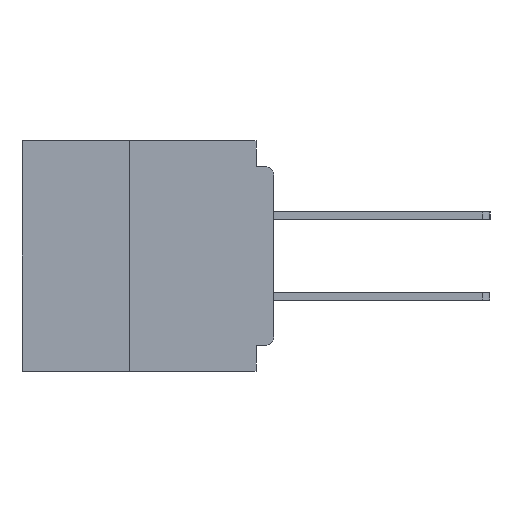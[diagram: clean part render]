
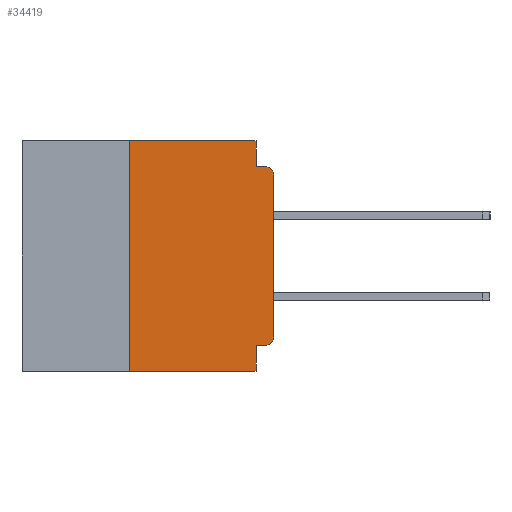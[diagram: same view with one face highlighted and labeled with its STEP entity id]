
A CAD part, left-side view. The second image highlights one B-rep face of the part: STEP entity #34419.
In plain terms, the highlighted planar face has unit normal (-1, 0, 0).
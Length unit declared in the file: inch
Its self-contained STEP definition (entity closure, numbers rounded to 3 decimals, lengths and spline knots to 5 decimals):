
#31 = VECTOR ( 'NONE', #66891, 39.37008 ) ;
#384 = VERTEX_POINT ( 'NONE', #27047 ) ;
#1747 = VERTEX_POINT ( 'NONE', #54699 ) ;
#2224 = DIRECTION ( 'NONE',  ( 0., 0., -1. ) ) ;
#2491 = LINE ( 'NONE', #56251, #28710 ) ;
#3141 = CARTESIAN_POINT ( 'NONE',  ( 0., 0.25, -0.4 ) ) ;
#3195 = DIRECTION ( 'NONE',  ( -1., 0., 0. ) ) ;
#5137 = CARTESIAN_POINT ( 'NONE',  ( 0., 0.031, -0.4 ) ) ;
#6063 = CARTESIAN_POINT ( 'NONE',  ( 0., 0., -0.355 ) ) ;
#6633 = DIRECTION ( 'NONE',  ( 0., -1., 0. ) ) ;
#8123 = EDGE_CURVE ( 'NONE', #63116, #41610, #60506, .T. ) ;
#8308 = ORIENTED_EDGE ( 'NONE', *, *, #26199, .F. ) ;
#9129 = VERTEX_POINT ( 'NONE', #14503 ) ;
#11056 = CIRCLE ( 'NONE', #36068, 0.015 ) ;
#11077 = LINE ( 'NONE', #55611, #64418 ) ;
#11372 = DIRECTION ( 'NONE',  ( 0., 1., 0. ) ) ;
#11818 = CARTESIAN_POINT ( 'NONE',  ( 0., 0.031, -0.4 ) ) ;
#12473 = CIRCLE ( 'NONE', #44600, 0.015 ) ;
#12802 = VECTOR ( 'NONE', #41342, 39.37008 ) ;
#13586 = ORIENTED_EDGE ( 'NONE', *, *, #39826, .F. ) ;
#14503 = CARTESIAN_POINT ( 'NONE',  ( 0., 0., -0.34 ) ) ;
#15498 = DIRECTION ( 'NONE',  ( 0., -1., 0. ) ) ;
#16225 = LINE ( 'NONE', #37921, #40651 ) ;
#16384 = ORIENTED_EDGE ( 'NONE', *, *, #24180, .T. ) ;
#16412 = VECTOR ( 'NONE', #15498, 39.37008 ) ;
#17131 = EDGE_LOOP ( 'NONE', ( #53732, #59925, #13586, #56914, #32302, #30323, #16384, #34218, #8308, #52899 ) ) ;
#19761 = DIRECTION ( 'NONE',  ( 0., 0., 1. ) ) ;
#20773 = EDGE_CURVE ( 'NONE', #53980, #32496, #11077, .T. ) ;
#24178 = VERTEX_POINT ( 'NONE', #46769 ) ;
#24180 = EDGE_CURVE ( 'NONE', #53980, #41610, #30294, .T. ) ;
#24977 = PLANE ( 'NONE',  #39790 ) ;
#26199 = EDGE_CURVE ( 'NONE', #1747, #63116, #34080, .T. ) ;
#27047 = CARTESIAN_POINT ( 'NONE',  ( 0., 0., -0.06 ) ) ;
#28710 = VECTOR ( 'NONE', #61418, 39.37008 ) ;
#30294 = LINE ( 'NONE', #67096, #16412 ) ;
#30323 = ORIENTED_EDGE ( 'NONE', *, *, #20773, .F. ) ;
#30913 = CARTESIAN_POINT ( 'NONE',  ( 0., 0., 0. ) ) ;
#31245 = VERTEX_POINT ( 'NONE', #44034 ) ;
#32302 = ORIENTED_EDGE ( 'NONE', *, *, #44578, .F. ) ;
#32496 = VERTEX_POINT ( 'NONE', #35422 ) ;
#32910 = EDGE_CURVE ( 'NONE', #1747, #9129, #11056, .T. ) ;
#33536 = DIRECTION ( 'NONE',  ( -1., 0., 0. ) ) ;
#33769 = CARTESIAN_POINT ( 'NONE',  ( 0., 0.015, -0.045 ) ) ;
#34080 = LINE ( 'NONE', #6063, #58157 ) ;
#34218 = ORIENTED_EDGE ( 'NONE', *, *, #8123, .F. ) ;
#34419 = ADVANCED_FACE ( 'NONE', ( #49069 ), #24977, .F. ) ;
#34508 = CARTESIAN_POINT ( 'NONE',  ( 0., 0.015, -0.06 ) ) ;
#35411 = DIRECTION ( 'NONE',  ( 0., 0., -1. ) ) ;
#35422 = CARTESIAN_POINT ( 'NONE',  ( 0., 0.25, 0. ) ) ;
#35795 = EDGE_CURVE ( 'NONE', #24178, #31245, #65696, .T. ) ;
#36068 = AXIS2_PLACEMENT_3D ( 'NONE', #64267, #33536, #2224 ) ;
#36228 = CARTESIAN_POINT ( 'NONE',  ( 0., 0.031, 0. ) ) ;
#37822 = DIRECTION ( 'NONE',  ( 0., 0., -1. ) ) ;
#37921 = CARTESIAN_POINT ( 'NONE',  ( 0., 0., -0.045 ) ) ;
#39737 = DIRECTION ( 'NONE',  ( 0., 0., -1. ) ) ;
#39790 = AXIS2_PLACEMENT_3D ( 'NONE', #60965, #66092, #35411 ) ;
#39826 = EDGE_CURVE ( 'NONE', #31245, #44933, #16225, .T. ) ;
#40523 = LINE ( 'NONE', #30913, #12802 ) ;
#40651 = VECTOR ( 'NONE', #6633, 39.37008 ) ;
#41342 = DIRECTION ( 'NONE',  ( 0., 0., 1. ) ) ;
#41610 = VERTEX_POINT ( 'NONE', #5137 ) ;
#44034 = CARTESIAN_POINT ( 'NONE',  ( 0., 0.031, -0.045 ) ) ;
#44578 = EDGE_CURVE ( 'NONE', #32496, #24178, #2491, .T. ) ;
#44600 = AXIS2_PLACEMENT_3D ( 'NONE', #34508, #3195, #39737 ) ;
#44933 = VERTEX_POINT ( 'NONE', #33769 ) ;
#46316 = EDGE_CURVE ( 'NONE', #384, #44933, #12473, .T. ) ;
#46769 = CARTESIAN_POINT ( 'NONE',  ( 0., 0.031, 0. ) ) ;
#49069 = FACE_OUTER_BOUND ( 'NONE', #17131, .T. ) ;
#49655 = EDGE_CURVE ( 'NONE', #9129, #384, #40523, .T. ) ;
#52899 = ORIENTED_EDGE ( 'NONE', *, *, #32910, .T. ) ;
#53732 = ORIENTED_EDGE ( 'NONE', *, *, #49655, .T. ) ;
#53859 = CARTESIAN_POINT ( 'NONE',  ( 0., 0.031, -0.355 ) ) ;
#53980 = VERTEX_POINT ( 'NONE', #3141 ) ;
#54699 = CARTESIAN_POINT ( 'NONE',  ( 0., 0.015, -0.355 ) ) ;
#55611 = CARTESIAN_POINT ( 'NONE',  ( 0., 0.25, -0.4 ) ) ;
#56251 = CARTESIAN_POINT ( 'NONE',  ( 0., 0.437, 0. ) ) ;
#56914 = ORIENTED_EDGE ( 'NONE', *, *, #35795, .F. ) ;
#57266 = VECTOR ( 'NONE', #37822, 39.37008 ) ;
#58157 = VECTOR ( 'NONE', #11372, 39.37008 ) ;
#59925 = ORIENTED_EDGE ( 'NONE', *, *, #46316, .T. ) ;
#60506 = LINE ( 'NONE', #11818, #57266 ) ;
#60965 = CARTESIAN_POINT ( 'NONE',  ( 0., 0.437, 0. ) ) ;
#61418 = DIRECTION ( 'NONE',  ( 0., -1., 0. ) ) ;
#63116 = VERTEX_POINT ( 'NONE', #53859 ) ;
#64267 = CARTESIAN_POINT ( 'NONE',  ( 0., 0.015, -0.34 ) ) ;
#64418 = VECTOR ( 'NONE', #19761, 39.37008 ) ;
#65696 = LINE ( 'NONE', #36228, #31 ) ;
#66092 = DIRECTION ( 'NONE',  ( 1., 0., 0. ) ) ;
#66891 = DIRECTION ( 'NONE',  ( 0., 0., -1. ) ) ;
#67096 = CARTESIAN_POINT ( 'NONE',  ( 0., 0.437, -0.4 ) ) ;
